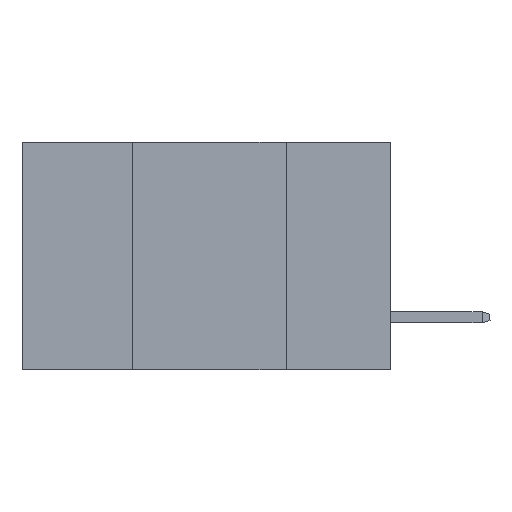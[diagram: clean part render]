
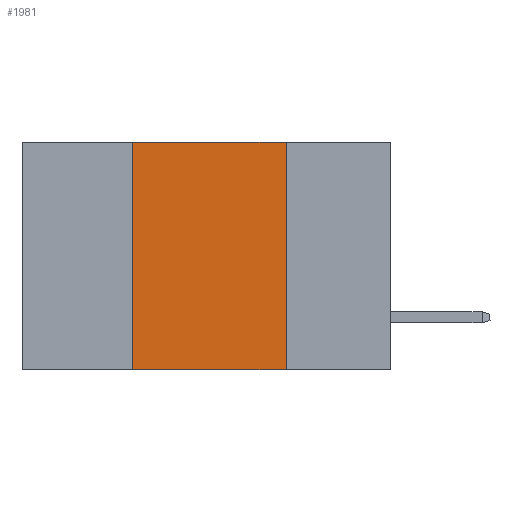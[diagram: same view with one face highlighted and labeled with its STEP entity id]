
A CAD part, left-side view. The second image highlights one B-rep face of the part: STEP entity #1981.
In plain terms, the highlighted planar face has unit normal (-1, 0, 0).
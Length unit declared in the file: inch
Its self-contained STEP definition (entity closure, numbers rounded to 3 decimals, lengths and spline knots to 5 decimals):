
#250 = EDGE_CURVE ( 'NONE', #12035, #11765, #3453, .T. ) ;
#572 = ORIENTED_EDGE ( 'NONE', *, *, #9161, .T. ) ;
#1981 = ADVANCED_FACE ( 'NONE', ( #5136 ), #11273, .F. ) ;
#2087 = DIRECTION ( 'NONE',  ( 0., -1., 0. ) ) ;
#2417 = CARTESIAN_POINT ( 'NONE',  ( 0., 0.42, -0.37 ) ) ;
#2737 = CARTESIAN_POINT ( 'NONE',  ( 0., 0.17, 0. ) ) ;
#2859 = DIRECTION ( 'NONE',  ( 0., 0., -1. ) ) ;
#3453 = LINE ( 'NONE', #2737, #15089 ) ;
#3633 = VERTEX_POINT ( 'NONE', #2417 ) ;
#4597 = CARTESIAN_POINT ( 'NONE',  ( 0., 0.17, -0.37 ) ) ;
#4943 = EDGE_LOOP ( 'NONE', ( #7234, #10978, #14732, #572 ) ) ;
#5136 = FACE_OUTER_BOUND ( 'NONE', #4943, .T. ) ;
#5359 = LINE ( 'NONE', #9074, #9056 ) ;
#6107 = AXIS2_PLACEMENT_3D ( 'NONE', #16584, #10766, #10210 ) ;
#6802 = LINE ( 'NONE', #14018, #10074 ) ;
#7234 = ORIENTED_EDGE ( 'NONE', *, *, #250, .F. ) ;
#8733 = LINE ( 'NONE', #10258, #15775 ) ;
#9056 = VECTOR ( 'NONE', #2087, 39.37008 ) ;
#9074 = CARTESIAN_POINT ( 'NONE',  ( 0., 0.6, -0.37 ) ) ;
#9161 = EDGE_CURVE ( 'NONE', #3633, #11765, #5359, .T. ) ;
#9925 = VERTEX_POINT ( 'NONE', #14619 ) ;
#10074 = VECTOR ( 'NONE', #11169, 39.37008 ) ;
#10210 = DIRECTION ( 'NONE',  ( 0., 0., -1. ) ) ;
#10258 = CARTESIAN_POINT ( 'NONE',  ( 0., 0.42, 0. ) ) ;
#10766 = DIRECTION ( 'NONE',  ( 1., 0., 0. ) ) ;
#10978 = ORIENTED_EDGE ( 'NONE', *, *, #11579, .F. ) ;
#11169 = DIRECTION ( 'NONE',  ( 0., -1., 0. ) ) ;
#11273 = PLANE ( 'NONE',  #6107 ) ;
#11579 = EDGE_CURVE ( 'NONE', #9925, #12035, #6802, .T. ) ;
#11765 = VERTEX_POINT ( 'NONE', #4597 ) ;
#12035 = VERTEX_POINT ( 'NONE', #15275 ) ;
#14018 = CARTESIAN_POINT ( 'NONE',  ( 0., 0.6, 0. ) ) ;
#14619 = CARTESIAN_POINT ( 'NONE',  ( 0., 0.42, 0. ) ) ;
#14732 = ORIENTED_EDGE ( 'NONE', *, *, #14858, .F. ) ;
#14858 = EDGE_CURVE ( 'NONE', #3633, #9925, #8733, .T. ) ;
#15089 = VECTOR ( 'NONE', #2859, 39.37008 ) ;
#15275 = CARTESIAN_POINT ( 'NONE',  ( 0., 0.17, 0. ) ) ;
#15775 = VECTOR ( 'NONE', #17219, 39.37008 ) ;
#16584 = CARTESIAN_POINT ( 'NONE',  ( 0., 0.6, 0. ) ) ;
#17219 = DIRECTION ( 'NONE',  ( 0., 0., 1. ) ) ;
